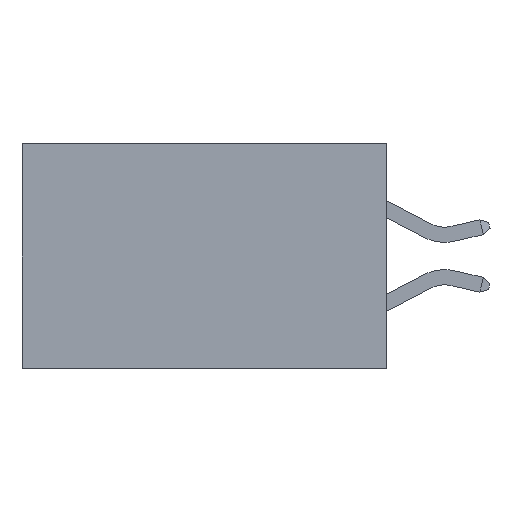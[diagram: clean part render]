
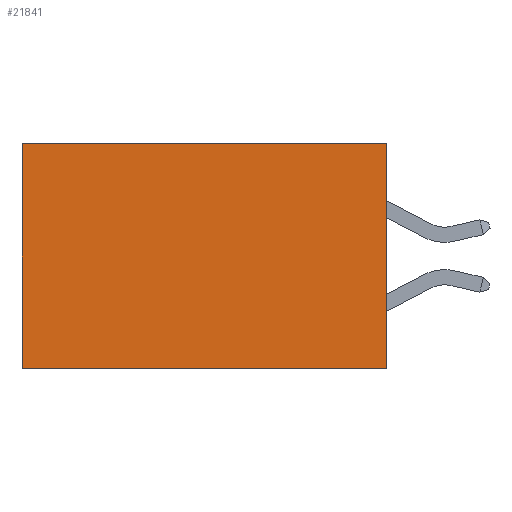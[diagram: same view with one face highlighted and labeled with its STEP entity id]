
A CAD part, left-side view. The second image highlights one B-rep face of the part: STEP entity #21841.
In plain terms, the highlighted planar face has unit normal (-1, 0, 0).
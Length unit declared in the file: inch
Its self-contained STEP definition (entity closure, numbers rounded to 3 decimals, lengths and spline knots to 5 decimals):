
#1511 = ORIENTED_EDGE ( 'NONE', *, *, #4505, .T. ) ;
#1840 = LINE ( 'NONE', #8590, #16359 ) ;
#1995 = LINE ( 'NONE', #15234, #12892 ) ;
#2431 = VERTEX_POINT ( 'NONE', #9925 ) ;
#2591 = VECTOR ( 'NONE', #21419, 39.37008 ) ;
#4292 = CARTESIAN_POINT ( 'NONE',  ( 0.2615, 0., -0.37 ) ) ;
#4409 = CARTESIAN_POINT ( 'NONE',  ( 0.2615, 0., -0.37 ) ) ;
#4505 = EDGE_CURVE ( 'NONE', #18243, #2431, #1840, .T. ) ;
#4694 = PLANE ( 'NONE',  #15970 ) ;
#5201 = FACE_OUTER_BOUND ( 'NONE', #13324, .T. ) ;
#7826 = LINE ( 'NONE', #4292, #20581 ) ;
#8590 = CARTESIAN_POINT ( 'NONE',  ( 0.2615, 0., 0. ) ) ;
#8797 = ORIENTED_EDGE ( 'NONE', *, *, #13386, .T. ) ;
#9270 = DIRECTION ( 'NONE',  ( 0., 0., -1. ) ) ;
#9925 = CARTESIAN_POINT ( 'NONE',  ( 0.2615, 0.6, 0. ) ) ;
#10410 = VERTEX_POINT ( 'NONE', #4409 ) ;
#11409 = ORIENTED_EDGE ( 'NONE', *, *, #16047, .F. ) ;
#11433 = CARTESIAN_POINT ( 'NONE',  ( 0.2615, 0., -0.37 ) ) ;
#11742 = LINE ( 'NONE', #14627, #2591 ) ;
#12157 = EDGE_CURVE ( 'NONE', #18243, #10410, #7826, .T. ) ;
#12892 = VECTOR ( 'NONE', #13905, 39.37008 ) ;
#13324 = EDGE_LOOP ( 'NONE', ( #8797, #11409, #19590, #1511 ) ) ;
#13386 = EDGE_CURVE ( 'NONE', #2431, #20141, #11742, .T. ) ;
#13905 = DIRECTION ( 'NONE',  ( 0., 1., 0. ) ) ;
#14262 = CARTESIAN_POINT ( 'NONE',  ( 0.2615, 0.6, -0.37 ) ) ;
#14627 = CARTESIAN_POINT ( 'NONE',  ( 0.2615, 0.6, -0.37 ) ) ;
#14948 = DIRECTION ( 'NONE',  ( 1., 0., 0. ) ) ;
#15234 = CARTESIAN_POINT ( 'NONE',  ( 0.2615, 0., -0.37 ) ) ;
#15970 = AXIS2_PLACEMENT_3D ( 'NONE', #11433, #14948, #18182 ) ;
#16047 = EDGE_CURVE ( 'NONE', #10410, #20141, #1995, .T. ) ;
#16359 = VECTOR ( 'NONE', #17100, 39.37008 ) ;
#17100 = DIRECTION ( 'NONE',  ( 0., 1., 0. ) ) ;
#18182 = DIRECTION ( 'NONE',  ( 0., 0., -1. ) ) ;
#18243 = VERTEX_POINT ( 'NONE', #18351 ) ;
#18351 = CARTESIAN_POINT ( 'NONE',  ( 0.2615, 0., 0. ) ) ;
#19590 = ORIENTED_EDGE ( 'NONE', *, *, #12157, .F. ) ;
#20141 = VERTEX_POINT ( 'NONE', #14262 ) ;
#20581 = VECTOR ( 'NONE', #9270, 39.37008 ) ;
#21419 = DIRECTION ( 'NONE',  ( 0., 0., -1. ) ) ;
#21841 = ADVANCED_FACE ( 'NONE', ( #5201 ), #4694, .F. ) ;
